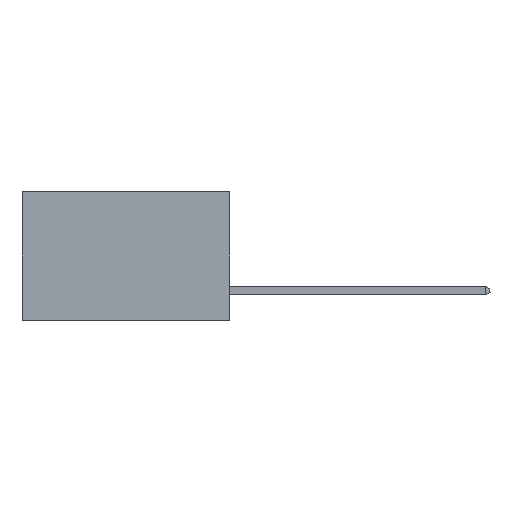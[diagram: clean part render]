
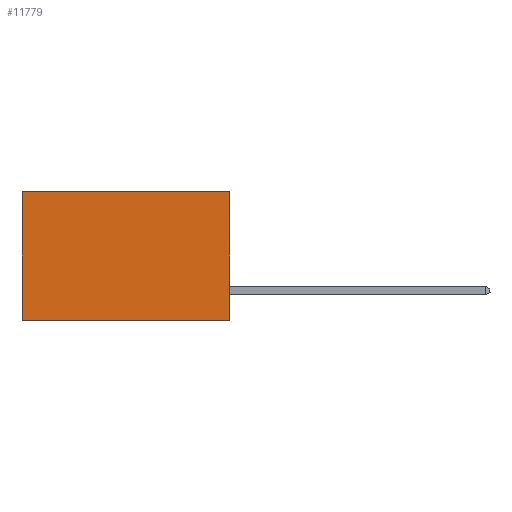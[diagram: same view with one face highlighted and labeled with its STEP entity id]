
A CAD part, left-side view. The second image highlights one B-rep face of the part: STEP entity #11779.
In plain terms, the highlighted planar face has unit normal (-1, 0, 0).
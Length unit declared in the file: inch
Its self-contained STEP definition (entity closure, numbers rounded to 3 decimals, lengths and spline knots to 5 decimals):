
#29 = PLANE ( 'NONE',  #11966 ) ;
#416 = VERTEX_POINT ( 'NONE', #10445 ) ;
#1256 = LINE ( 'NONE', #12588, #8229 ) ;
#1566 = DIRECTION ( 'NONE',  ( 0., 1., 0. ) ) ;
#3117 = CARTESIAN_POINT ( 'NONE',  ( 0.298, 0., 0. ) ) ;
#3358 = VERTEX_POINT ( 'NONE', #10668 ) ;
#4157 = EDGE_CURVE ( 'NONE', #416, #18977, #1256, .T. ) ;
#4164 = CARTESIAN_POINT ( 'NONE',  ( 0.298, 0.6, 0. ) ) ;
#4562 = ORIENTED_EDGE ( 'NONE', *, *, #15969, .T. ) ;
#5019 = ORIENTED_EDGE ( 'NONE', *, *, #4157, .T. ) ;
#5265 = VERTEX_POINT ( 'NONE', #5629 ) ;
#5629 = CARTESIAN_POINT ( 'NONE',  ( 0.298, 0.6, -0.37 ) ) ;
#5865 = EDGE_CURVE ( 'NONE', #3358, #5265, #19199, .T. ) ;
#6040 = CARTESIAN_POINT ( 'NONE',  ( 0.298, 0., -0.37 ) ) ;
#6407 = DIRECTION ( 'NONE',  ( 0., 0., -1. ) ) ;
#7938 = LINE ( 'NONE', #18416, #13953 ) ;
#7976 = EDGE_CURVE ( 'NONE', #416, #3358, #17015, .T. ) ;
#8229 = VECTOR ( 'NONE', #14199, 39.37008 ) ;
#8673 = VECTOR ( 'NONE', #18933, 39.37008 ) ;
#10019 = ORIENTED_EDGE ( 'NONE', *, *, #7976, .F. ) ;
#10445 = CARTESIAN_POINT ( 'NONE',  ( 0.298, 0., 0. ) ) ;
#10668 = CARTESIAN_POINT ( 'NONE',  ( 0.298, 0., -0.37 ) ) ;
#11779 = ADVANCED_FACE ( 'NONE', ( #15668 ), #29, .F. ) ;
#11966 = AXIS2_PLACEMENT_3D ( 'NONE', #3117, #18490, #6407 ) ;
#12588 = CARTESIAN_POINT ( 'NONE',  ( 0.298, 0., 0. ) ) ;
#13658 = VECTOR ( 'NONE', #1566, 39.37008 ) ;
#13953 = VECTOR ( 'NONE', #19697, 39.37008 ) ;
#14199 = DIRECTION ( 'NONE',  ( 0., 1., 0. ) ) ;
#14347 = CARTESIAN_POINT ( 'NONE',  ( 0.298, 0., 0. ) ) ;
#14406 = EDGE_LOOP ( 'NONE', ( #4562, #18368, #10019, #5019 ) ) ;
#15668 = FACE_OUTER_BOUND ( 'NONE', #14406, .T. ) ;
#15969 = EDGE_CURVE ( 'NONE', #18977, #5265, #7938, .T. ) ;
#17015 = LINE ( 'NONE', #14347, #8673 ) ;
#18368 = ORIENTED_EDGE ( 'NONE', *, *, #5865, .F. ) ;
#18416 = CARTESIAN_POINT ( 'NONE',  ( 0.298, 0.6, 0. ) ) ;
#18490 = DIRECTION ( 'NONE',  ( 1., 0., 0. ) ) ;
#18933 = DIRECTION ( 'NONE',  ( 0., 0., -1. ) ) ;
#18977 = VERTEX_POINT ( 'NONE', #4164 ) ;
#19199 = LINE ( 'NONE', #6040, #13658 ) ;
#19697 = DIRECTION ( 'NONE',  ( 0., 0., -1. ) ) ;
